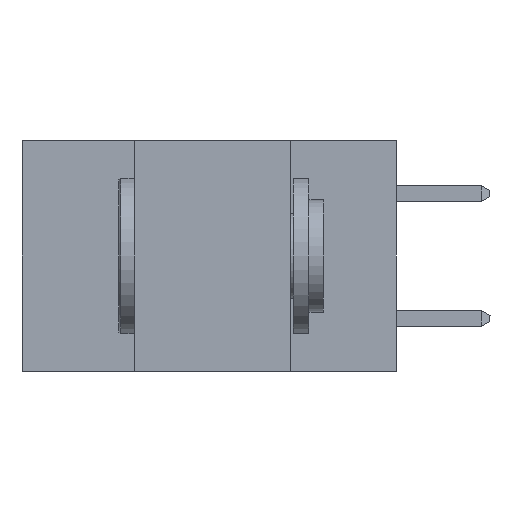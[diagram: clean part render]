
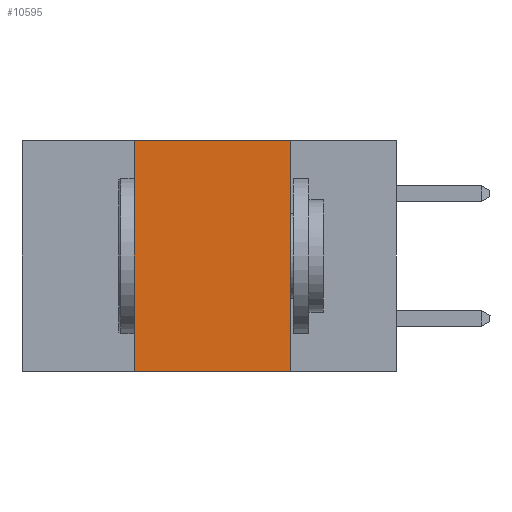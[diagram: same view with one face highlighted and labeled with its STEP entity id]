
A CAD part, left-side view. The second image highlights one B-rep face of the part: STEP entity #10595.
In plain terms, the highlighted planar face has unit normal (-1, 0, 0).
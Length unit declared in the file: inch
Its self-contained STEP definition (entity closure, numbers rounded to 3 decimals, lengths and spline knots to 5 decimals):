
#575 = LINE ( 'NONE', #11141, #9245 ) ;
#702 = FACE_OUTER_BOUND ( 'NONE', #7835, .T. ) ;
#1607 = VERTEX_POINT ( 'NONE', #9616 ) ;
#2381 = VERTEX_POINT ( 'NONE', #8012 ) ;
#2856 = CARTESIAN_POINT ( 'NONE',  ( 0., 0.17, -0.37 ) ) ;
#4245 = DIRECTION ( 'NONE',  ( 0., -1., 0. ) ) ;
#4414 = DIRECTION ( 'NONE',  ( 0., 0., 1. ) ) ;
#4519 = CARTESIAN_POINT ( 'NONE',  ( 0., 0.42, -0.37 ) ) ;
#5059 = VECTOR ( 'NONE', #12090, 39.37008 ) ;
#5321 = ORIENTED_EDGE ( 'NONE', *, *, #12919, .F. ) ;
#5337 = VERTEX_POINT ( 'NONE', #7383 ) ;
#6934 = EDGE_CURVE ( 'NONE', #2381, #14887, #11614, .T. ) ;
#7383 = CARTESIAN_POINT ( 'NONE',  ( 0., 0.42, -0.37 ) ) ;
#7797 = VECTOR ( 'NONE', #11003, 39.37008 ) ;
#7835 = EDGE_LOOP ( 'NONE', ( #8558, #5321, #9003, #8491 ) ) ;
#8012 = CARTESIAN_POINT ( 'NONE',  ( 0., 0.17, 0. ) ) ;
#8324 = CARTESIAN_POINT ( 'NONE',  ( 0., 0.6, 0. ) ) ;
#8491 = ORIENTED_EDGE ( 'NONE', *, *, #14274, .T. ) ;
#8558 = ORIENTED_EDGE ( 'NONE', *, *, #6934, .F. ) ;
#8925 = DIRECTION ( 'NONE',  ( 0., 0., -1. ) ) ;
#9003 = ORIENTED_EDGE ( 'NONE', *, *, #13579, .F. ) ;
#9078 = LINE ( 'NONE', #4519, #12537 ) ;
#9245 = VECTOR ( 'NONE', #4245, 39.37008 ) ;
#9465 = DIRECTION ( 'NONE',  ( 1., 0., 0. ) ) ;
#9522 = PLANE ( 'NONE',  #11929 ) ;
#9616 = CARTESIAN_POINT ( 'NONE',  ( 0., 0.42, 0. ) ) ;
#10588 = CARTESIAN_POINT ( 'NONE',  ( 0., 0.6, 0. ) ) ;
#10595 = ADVANCED_FACE ( 'NONE', ( #702 ), #9522, .F. ) ;
#11003 = DIRECTION ( 'NONE',  ( 0., -1., 0. ) ) ;
#11141 = CARTESIAN_POINT ( 'NONE',  ( 0., 0.6, -0.37 ) ) ;
#11278 = LINE ( 'NONE', #10588, #7797 ) ;
#11614 = LINE ( 'NONE', #12162, #5059 ) ;
#11929 = AXIS2_PLACEMENT_3D ( 'NONE', #8324, #9465, #8925 ) ;
#12090 = DIRECTION ( 'NONE',  ( 0., 0., -1. ) ) ;
#12162 = CARTESIAN_POINT ( 'NONE',  ( 0., 0.17, -0.37 ) ) ;
#12537 = VECTOR ( 'NONE', #4414, 39.37008 ) ;
#12919 = EDGE_CURVE ( 'NONE', #1607, #2381, #11278, .T. ) ;
#13579 = EDGE_CURVE ( 'NONE', #5337, #1607, #9078, .T. ) ;
#14274 = EDGE_CURVE ( 'NONE', #5337, #14887, #575, .T. ) ;
#14887 = VERTEX_POINT ( 'NONE', #2856 ) ;
